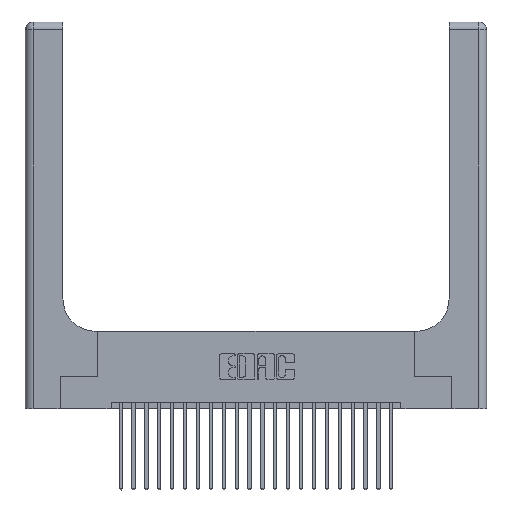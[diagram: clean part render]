
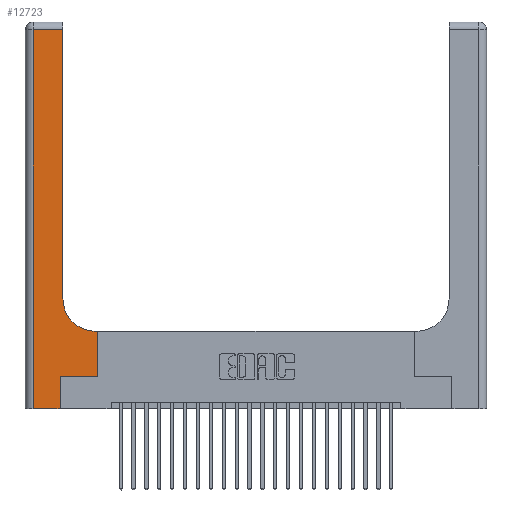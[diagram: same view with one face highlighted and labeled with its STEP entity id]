
A CAD part, top view. The second image highlights one B-rep face of the part: STEP entity #12723.
In plain terms, the highlighted planar face has unit normal (0, 0, 1).
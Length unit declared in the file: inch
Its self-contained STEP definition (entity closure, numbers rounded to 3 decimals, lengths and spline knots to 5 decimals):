
#1325 = DIRECTION ( 'NONE',  ( 1., 0., 0. ) ) ;
#1784 = ORIENTED_EDGE ( 'NONE', *, *, #4257, .T. ) ;
#1832 = CARTESIAN_POINT ( 'NONE',  ( 0.06, 3., 0.37 ) ) ;
#1872 = VECTOR ( 'NONE', #20920, 39.37008 ) ;
#1883 = CARTESIAN_POINT ( 'NONE',  ( 0.5415, 0.6, 0.37 ) ) ;
#2110 = PLANE ( 'NONE',  #23529 ) ;
#2943 = CIRCLE ( 'NONE', #13854, 0.25 ) ;
#3100 = CARTESIAN_POINT ( 'NONE',  ( 0.269, 0., 0.37 ) ) ;
#3416 = CARTESIAN_POINT ( 'NONE',  ( 0., 2.94, 0.37 ) ) ;
#3668 = VECTOR ( 'NONE', #6955, 39.37008 ) ;
#4257 = EDGE_CURVE ( 'NONE', #17828, #18361, #24817, .T. ) ;
#4688 = CARTESIAN_POINT ( 'NONE',  ( 0.5585, 0.25, 0.37 ) ) ;
#4780 = VERTEX_POINT ( 'NONE', #13479 ) ;
#4934 = LINE ( 'NONE', #1832, #8859 ) ;
#5274 = CARTESIAN_POINT ( 'NONE',  ( 0.5585, 0.6, 0.37 ) ) ;
#5434 = VERTEX_POINT ( 'NONE', #12531 ) ;
#5632 = LINE ( 'NONE', #18225, #16278 ) ;
#6238 = EDGE_CURVE ( 'NONE', #22318, #22379, #4934, .T. ) ;
#6955 = DIRECTION ( 'NONE',  ( 0., 1., 0. ) ) ;
#8639 = LINE ( 'NONE', #18340, #23604 ) ;
#8754 = LINE ( 'NONE', #19719, #12729 ) ;
#8859 = VECTOR ( 'NONE', #17322, 39.37008 ) ;
#9566 = EDGE_CURVE ( 'NONE', #9576, #5434, #2943, .T. ) ;
#9576 = VERTEX_POINT ( 'NONE', #1883 ) ;
#9934 = CARTESIAN_POINT ( 'NONE',  ( 0.06, 2.94, 0.37 ) ) ;
#10010 = DIRECTION ( 'NONE',  ( 0., 0., -1. ) ) ;
#11333 = EDGE_CURVE ( 'NONE', #12263, #4780, #24944, .T. ) ;
#12263 = VERTEX_POINT ( 'NONE', #15515 ) ;
#12531 = CARTESIAN_POINT ( 'NONE',  ( 0.2915, 0.85, 0.37 ) ) ;
#12723 = ADVANCED_FACE ( 'NONE', ( #22133 ), #2110, .F. ) ;
#12729 = VECTOR ( 'NONE', #23793, 39.37008 ) ;
#13226 = DIRECTION ( 'NONE',  ( 0., 0., -1. ) ) ;
#13479 = CARTESIAN_POINT ( 'NONE',  ( 0.269, 0.25, 0.37 ) ) ;
#13615 = CARTESIAN_POINT ( 'NONE',  ( 0.5585, 0.25, 0.37 ) ) ;
#13854 = AXIS2_PLACEMENT_3D ( 'NONE', #17212, #13226, #1325 ) ;
#14585 = DIRECTION ( 'NONE',  ( 1., 0., 0. ) ) ;
#15515 = CARTESIAN_POINT ( 'NONE',  ( 0.269, 0., 0.37 ) ) ;
#15949 = ORIENTED_EDGE ( 'NONE', *, *, #22794, .T. ) ;
#16278 = VECTOR ( 'NONE', #14585, 39.37008 ) ;
#16475 = EDGE_CURVE ( 'NONE', #22379, #12263, #20138, .T. ) ;
#16581 = DIRECTION ( 'NONE',  ( 1., 0., 0. ) ) ;
#16995 = EDGE_LOOP ( 'NONE', ( #24960, #17155, #20315, #18294, #22282, #19949, #1784, #15949, #19739 ) ) ;
#17155 = ORIENTED_EDGE ( 'NONE', *, *, #24587, .T. ) ;
#17212 = CARTESIAN_POINT ( 'NONE',  ( 0.5415, 0.85, 0.37 ) ) ;
#17322 = DIRECTION ( 'NONE',  ( 0., -1., 0. ) ) ;
#17513 = CARTESIAN_POINT ( 'NONE',  ( 0., 3., 0.37 ) ) ;
#17733 = DIRECTION ( 'NONE',  ( 0., 1., 0. ) ) ;
#17756 = CARTESIAN_POINT ( 'NONE',  ( 0.06, 0., 0.37 ) ) ;
#17828 = VERTEX_POINT ( 'NONE', #13615 ) ;
#18171 = EDGE_CURVE ( 'NONE', #5434, #20063, #8639, .T. ) ;
#18225 = CARTESIAN_POINT ( 'NONE',  ( 0.269, 0.25, 0.37 ) ) ;
#18294 = ORIENTED_EDGE ( 'NONE', *, *, #16475, .T. ) ;
#18340 = CARTESIAN_POINT ( 'NONE',  ( 0.2915, 3., 0.37 ) ) ;
#18361 = VERTEX_POINT ( 'NONE', #5274 ) ;
#18825 = EDGE_CURVE ( 'NONE', #4780, #17828, #5632, .T. ) ;
#19028 = VECTOR ( 'NONE', #17733, 39.37008 ) ;
#19671 = DIRECTION ( 'NONE',  ( -1., 0., 0. ) ) ;
#19719 = CARTESIAN_POINT ( 'NONE',  ( 0.2915, 0.6, 0.37 ) ) ;
#19739 = ORIENTED_EDGE ( 'NONE', *, *, #9566, .T. ) ;
#19949 = ORIENTED_EDGE ( 'NONE', *, *, #18825, .T. ) ;
#20063 = VERTEX_POINT ( 'NONE', #22235 ) ;
#20138 = LINE ( 'NONE', #22210, #22574 ) ;
#20315 = ORIENTED_EDGE ( 'NONE', *, *, #6238, .T. ) ;
#20920 = DIRECTION ( 'NONE',  ( -1., 0., 0. ) ) ;
#22133 = FACE_OUTER_BOUND ( 'NONE', #16995, .T. ) ;
#22195 = DIRECTION ( 'NONE',  ( 0., 1., 0. ) ) ;
#22210 = CARTESIAN_POINT ( 'NONE',  ( 0., 0., 0.37 ) ) ;
#22235 = CARTESIAN_POINT ( 'NONE',  ( 0.2915, 2.94, 0.37 ) ) ;
#22282 = ORIENTED_EDGE ( 'NONE', *, *, #11333, .T. ) ;
#22318 = VERTEX_POINT ( 'NONE', #9934 ) ;
#22379 = VERTEX_POINT ( 'NONE', #17756 ) ;
#22574 = VECTOR ( 'NONE', #16581, 39.37008 ) ;
#22794 = EDGE_CURVE ( 'NONE', #18361, #9576, #8754, .T. ) ;
#23529 = AXIS2_PLACEMENT_3D ( 'NONE', #17513, #10010, #19671 ) ;
#23604 = VECTOR ( 'NONE', #22195, 39.37008 ) ;
#23793 = DIRECTION ( 'NONE',  ( -1., 0., 0. ) ) ;
#24587 = EDGE_CURVE ( 'NONE', #20063, #22318, #24655, .T. ) ;
#24655 = LINE ( 'NONE', #3416, #1872 ) ;
#24817 = LINE ( 'NONE', #4688, #19028 ) ;
#24944 = LINE ( 'NONE', #3100, #3668 ) ;
#24960 = ORIENTED_EDGE ( 'NONE', *, *, #18171, .T. ) ;
